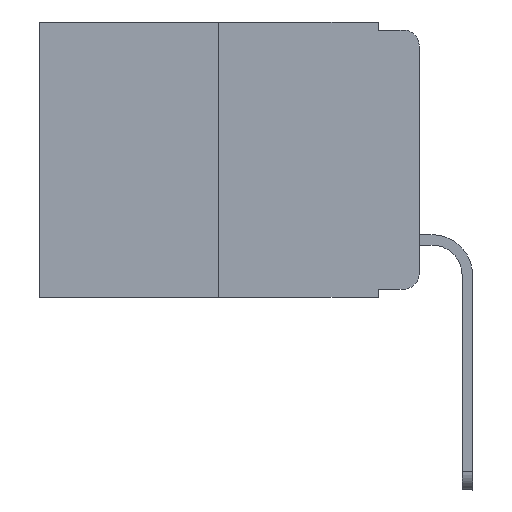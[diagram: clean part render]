
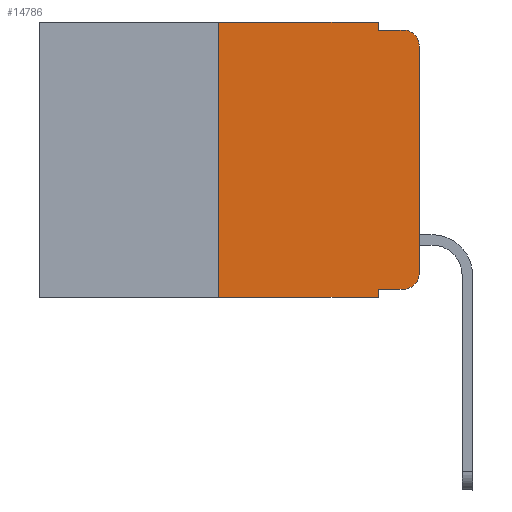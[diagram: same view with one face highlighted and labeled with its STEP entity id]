
A CAD part, left-side view. The second image highlights one B-rep face of the part: STEP entity #14786.
In plain terms, the highlighted planar face has unit normal (-1, 0, 0).
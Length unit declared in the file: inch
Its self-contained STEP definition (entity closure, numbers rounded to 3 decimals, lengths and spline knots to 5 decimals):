
#256 = DIRECTION ( 'NONE',  ( 0., -1., 0. ) ) ;
#359 = ORIENTED_EDGE ( 'NONE', *, *, #1068, .F. ) ;
#1065 = VERTEX_POINT ( 'NONE', #13039 ) ;
#1068 = EDGE_CURVE ( 'NONE', #19893, #11130, #11807, .T. ) ;
#1330 = DIRECTION ( 'NONE',  ( 0., 0., -1. ) ) ;
#1738 = CARTESIAN_POINT ( 'NONE',  ( 0., 0., 0. ) ) ;
#1859 = DIRECTION ( 'NONE',  ( 0., 0., 1. ) ) ;
#2202 = EDGE_CURVE ( 'NONE', #21992, #1065, #10686, .T. ) ;
#2222 = DIRECTION ( 'NONE',  ( 0., 0., -1. ) ) ;
#2703 = EDGE_CURVE ( 'NONE', #12779, #22654, #11272, .T. ) ;
#2739 = DIRECTION ( 'NONE',  ( 0., -1., 0. ) ) ;
#2865 = VECTOR ( 'NONE', #2739, 39.37008 ) ;
#3352 = PLANE ( 'NONE',  #9740 ) ;
#4156 = EDGE_CURVE ( 'NONE', #17457, #19893, #22595, .T. ) ;
#4223 = LINE ( 'NONE', #11523, #8247 ) ;
#4430 = CIRCLE ( 'NONE', #16864, 0.02 ) ;
#4586 = ORIENTED_EDGE ( 'NONE', *, *, #15267, .F. ) ;
#4657 = CARTESIAN_POINT ( 'NONE',  ( 0., 0.02, -0.313 ) ) ;
#4722 = CIRCLE ( 'NONE', #9624, 0.02 ) ;
#6430 = CARTESIAN_POINT ( 'NONE',  ( 0., 0.051, 0. ) ) ;
#6791 = VERTEX_POINT ( 'NONE', #17078 ) ;
#6890 = DIRECTION ( 'NONE',  ( 0., 0., 1. ) ) ;
#6943 = CARTESIAN_POINT ( 'NONE',  ( 0., 0.02, -0.01 ) ) ;
#7162 = VERTEX_POINT ( 'NONE', #17797 ) ;
#7176 = VECTOR ( 'NONE', #14938, 39.37008 ) ;
#7199 = CARTESIAN_POINT ( 'NONE',  ( 0., 0.473, 0. ) ) ;
#8247 = VECTOR ( 'NONE', #2222, 39.37008 ) ;
#8271 = DIRECTION ( 'NONE',  ( 0., -1., 0. ) ) ;
#8565 = DIRECTION ( 'NONE',  ( 0., 0., -1. ) ) ;
#8932 = VECTOR ( 'NONE', #6890, 39.37008 ) ;
#9253 = CARTESIAN_POINT ( 'NONE',  ( 0., 0.02, -0.333 ) ) ;
#9612 = ORIENTED_EDGE ( 'NONE', *, *, #2202, .T. ) ;
#9624 = AXIS2_PLACEMENT_3D ( 'NONE', #4657, #11837, #19044 ) ;
#9740 = AXIS2_PLACEMENT_3D ( 'NONE', #10529, #17712, #1330 ) ;
#9744 = EDGE_LOOP ( 'NONE', ( #9612, #10028, #359, #15084, #20227, #15158, #15916, #4586, #16732, #12100 ) ) ;
#9816 = VECTOR ( 'NONE', #1859, 39.37008 ) ;
#10028 = ORIENTED_EDGE ( 'NONE', *, *, #21827, .T. ) ;
#10529 = CARTESIAN_POINT ( 'NONE',  ( 0., 0.473, 0. ) ) ;
#10665 = EDGE_CURVE ( 'NONE', #7162, #17457, #21596, .T. ) ;
#10686 = LINE ( 'NONE', #1738, #9816 ) ;
#10806 = CARTESIAN_POINT ( 'NONE',  ( 0., 0., -0.313 ) ) ;
#11130 = VERTEX_POINT ( 'NONE', #6943 ) ;
#11142 = CARTESIAN_POINT ( 'NONE',  ( 0., 0.051, -0.01 ) ) ;
#11272 = LINE ( 'NONE', #14580, #7176 ) ;
#11523 = CARTESIAN_POINT ( 'NONE',  ( 0., 0.051, 0. ) ) ;
#11807 = LINE ( 'NONE', #11142, #20898 ) ;
#11837 = DIRECTION ( 'NONE',  ( -1., 0., 0. ) ) ;
#12100 = ORIENTED_EDGE ( 'NONE', *, *, #15931, .T. ) ;
#12779 = VERTEX_POINT ( 'NONE', #19204 ) ;
#13039 = CARTESIAN_POINT ( 'NONE',  ( 0., 0., -0.03 ) ) ;
#13276 = EDGE_CURVE ( 'NONE', #12779, #7162, #14555, .T. ) ;
#14285 = CARTESIAN_POINT ( 'NONE',  ( 0., 0.051, -0.01 ) ) ;
#14555 = LINE ( 'NONE', #23065, #8932 ) ;
#14580 = CARTESIAN_POINT ( 'NONE',  ( 0., 0.473, -0.343 ) ) ;
#14786 = ADVANCED_FACE ( 'NONE', ( #17477 ), #3352, .F. ) ;
#14938 = DIRECTION ( 'NONE',  ( 0., -1., 0. ) ) ;
#15084 = ORIENTED_EDGE ( 'NONE', *, *, #4156, .F. ) ;
#15158 = ORIENTED_EDGE ( 'NONE', *, *, #13276, .F. ) ;
#15231 = CARTESIAN_POINT ( 'NONE',  ( 0., 0.051, -0.333 ) ) ;
#15267 = EDGE_CURVE ( 'NONE', #6791, #22654, #4223, .T. ) ;
#15357 = CARTESIAN_POINT ( 'NONE',  ( 0., 0.051, -0.343 ) ) ;
#15916 = ORIENTED_EDGE ( 'NONE', *, *, #2703, .T. ) ;
#15931 = EDGE_CURVE ( 'NONE', #19092, #21992, #4722, .T. ) ;
#16673 = VECTOR ( 'NONE', #8565, 39.37008 ) ;
#16732 = ORIENTED_EDGE ( 'NONE', *, *, #19585, .T. ) ;
#16864 = AXIS2_PLACEMENT_3D ( 'NONE', #20960, #21194, #22723 ) ;
#16886 = LINE ( 'NONE', #15231, #2865 ) ;
#17078 = CARTESIAN_POINT ( 'NONE',  ( 0., 0.051, -0.333 ) ) ;
#17457 = VERTEX_POINT ( 'NONE', #22673 ) ;
#17477 = FACE_OUTER_BOUND ( 'NONE', #9744, .T. ) ;
#17712 = DIRECTION ( 'NONE',  ( 1., 0., 0. ) ) ;
#17797 = CARTESIAN_POINT ( 'NONE',  ( 0., 0.25, 0. ) ) ;
#18307 = VECTOR ( 'NONE', #256, 39.37008 ) ;
#19044 = DIRECTION ( 'NONE',  ( 0., 0., -1. ) ) ;
#19092 = VERTEX_POINT ( 'NONE', #9253 ) ;
#19204 = CARTESIAN_POINT ( 'NONE',  ( 0., 0.25, -0.343 ) ) ;
#19585 = EDGE_CURVE ( 'NONE', #6791, #19092, #16886, .T. ) ;
#19893 = VERTEX_POINT ( 'NONE', #14285 ) ;
#20227 = ORIENTED_EDGE ( 'NONE', *, *, #10665, .F. ) ;
#20898 = VECTOR ( 'NONE', #8271, 39.37008 ) ;
#20960 = CARTESIAN_POINT ( 'NONE',  ( 0., 0.02, -0.03 ) ) ;
#21194 = DIRECTION ( 'NONE',  ( -1., 0., 0. ) ) ;
#21596 = LINE ( 'NONE', #7199, #18307 ) ;
#21827 = EDGE_CURVE ( 'NONE', #1065, #11130, #4430, .T. ) ;
#21992 = VERTEX_POINT ( 'NONE', #10806 ) ;
#22595 = LINE ( 'NONE', #6430, #16673 ) ;
#22654 = VERTEX_POINT ( 'NONE', #15357 ) ;
#22673 = CARTESIAN_POINT ( 'NONE',  ( 0., 0.051, 0. ) ) ;
#22723 = DIRECTION ( 'NONE',  ( 0., 0., -1. ) ) ;
#23065 = CARTESIAN_POINT ( 'NONE',  ( 0., 0.25, 0. ) ) ;
